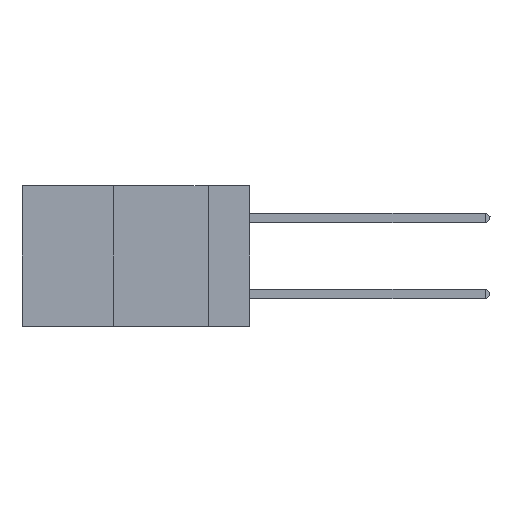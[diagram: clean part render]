
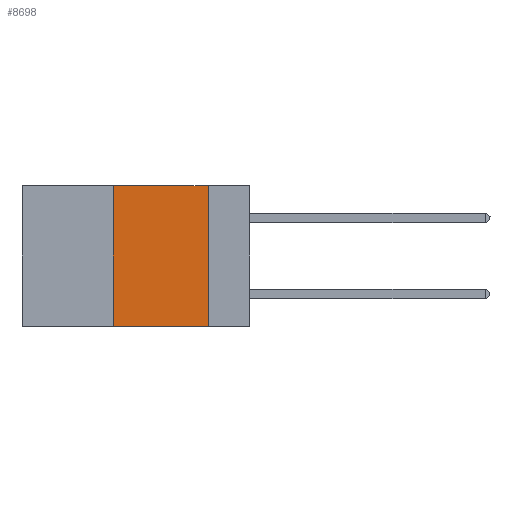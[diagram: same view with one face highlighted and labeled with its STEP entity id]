
A CAD part, left-side view. The second image highlights one B-rep face of the part: STEP entity #8698.
In plain terms, the highlighted planar face has unit normal (-1, 0, 0).
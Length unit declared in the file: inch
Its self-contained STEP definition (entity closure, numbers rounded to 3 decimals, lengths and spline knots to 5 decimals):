
#574 = CARTESIAN_POINT ( 'NONE',  ( 0., 0.36, 0. ) ) ;
#807 = LINE ( 'NONE', #574, #5509 ) ;
#922 = EDGE_CURVE ( 'NONE', #8134, #9295, #807, .T. ) ;
#1101 = PLANE ( 'NONE',  #5357 ) ;
#1359 = DIRECTION ( 'NONE',  ( 0., 0., 1. ) ) ;
#1628 = EDGE_CURVE ( 'NONE', #8134, #2442, #2349, .T. ) ;
#1902 = CARTESIAN_POINT ( 'NONE',  ( 0., 0.11, 0. ) ) ;
#2318 = CARTESIAN_POINT ( 'NONE',  ( 0., 0.11, 0. ) ) ;
#2349 = LINE ( 'NONE', #10917, #10648 ) ;
#2442 = VERTEX_POINT ( 'NONE', #4961 ) ;
#3317 = VECTOR ( 'NONE', #4958, 39.37008 ) ;
#3928 = EDGE_LOOP ( 'NONE', ( #8430, #8694, #11390, #4122 ) ) ;
#4026 = DIRECTION ( 'NONE',  ( 1., 0., 0. ) ) ;
#4077 = VECTOR ( 'NONE', #8253, 39.37008 ) ;
#4122 = ORIENTED_EDGE ( 'NONE', *, *, #1628, .T. ) ;
#4154 = EDGE_CURVE ( 'NONE', #4459, #2442, #10976, .T. ) ;
#4459 = VERTEX_POINT ( 'NONE', #2318 ) ;
#4958 = DIRECTION ( 'NONE',  ( 0., -1., 0. ) ) ;
#4961 = CARTESIAN_POINT ( 'NONE',  ( 0., 0.11, -0.37 ) ) ;
#4969 = CARTESIAN_POINT ( 'NONE',  ( 0., 0.36, -0.37 ) ) ;
#5357 = AXIS2_PLACEMENT_3D ( 'NONE', #7543, #4026, #10109 ) ;
#5509 = VECTOR ( 'NONE', #1359, 39.37008 ) ;
#5715 = LINE ( 'NONE', #8484, #3317 ) ;
#5826 = CARTESIAN_POINT ( 'NONE',  ( 0., 0.36, 0. ) ) ;
#6933 = FACE_OUTER_BOUND ( 'NONE', #3928, .T. ) ;
#7543 = CARTESIAN_POINT ( 'NONE',  ( 0., 0.6, 0. ) ) ;
#8134 = VERTEX_POINT ( 'NONE', #4969 ) ;
#8253 = DIRECTION ( 'NONE',  ( 0., 0., -1. ) ) ;
#8430 = ORIENTED_EDGE ( 'NONE', *, *, #4154, .F. ) ;
#8484 = CARTESIAN_POINT ( 'NONE',  ( 0., 0.6, 0. ) ) ;
#8694 = ORIENTED_EDGE ( 'NONE', *, *, #10791, .F. ) ;
#8698 = ADVANCED_FACE ( 'NONE', ( #6933 ), #1101, .F. ) ;
#9295 = VERTEX_POINT ( 'NONE', #5826 ) ;
#10109 = DIRECTION ( 'NONE',  ( 0., 0., -1. ) ) ;
#10387 = DIRECTION ( 'NONE',  ( 0., -1., 0. ) ) ;
#10648 = VECTOR ( 'NONE', #10387, 39.37008 ) ;
#10791 = EDGE_CURVE ( 'NONE', #9295, #4459, #5715, .T. ) ;
#10917 = CARTESIAN_POINT ( 'NONE',  ( 0., 0.6, -0.37 ) ) ;
#10976 = LINE ( 'NONE', #1902, #4077 ) ;
#11390 = ORIENTED_EDGE ( 'NONE', *, *, #922, .F. ) ;
